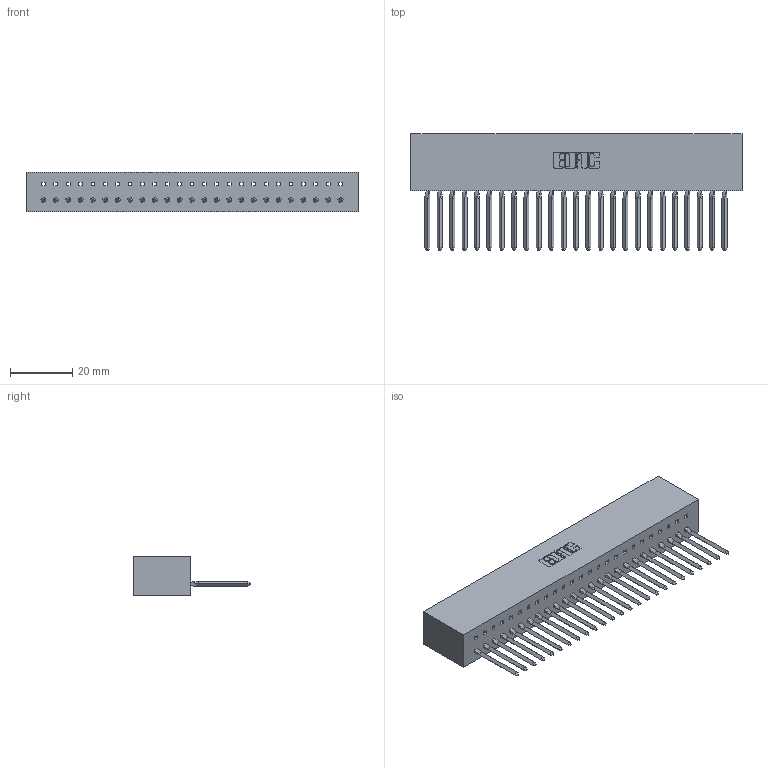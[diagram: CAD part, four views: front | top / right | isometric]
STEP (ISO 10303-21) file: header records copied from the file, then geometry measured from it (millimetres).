
FILE_DESCRIPTION (( 'STEP AP203' ), '1' );
FILE_NAME ('317-025-542-601.STEP', '2020-02-27T18:21:25', ( '' ), ( '' ), 'SwSTEP 2.0', 'SolidWorks 2016', '' );
FILE_SCHEMA (( 'CONFIG_CONTROL_DESIGN' ));
Length unit declared in the file: inch
Products named in the file (3): 317-025-542-601; 317 Part_Lugless; 317-290-003_542
Assembly tree (26 placements, depth 2):
  317-025-542-601
    317 Part_Lugless
    317-290-003_542  x25
Bounding box: 106.27 x 37.34 x 12.7 mm (x, y, z)
Volume: 17551 mm3; surface area: 21070 mm2
Topology: 26 solids, 26 shells, 1965 faces, 5664 edges, 3658 vertices
Faces by surface type: plane 1650, cylinder 215, bspline 100
Entity records: 36317 total; most frequent: CARTESIAN_POINT 6696, ORIENTED_EDGE 6384, DIRECTION 5342, EDGE_CURVE 3192, VECTOR 3030, LINE 3030, VERTEX_POINT 2122, AXIS2_PLACEMENT_3D 1156
